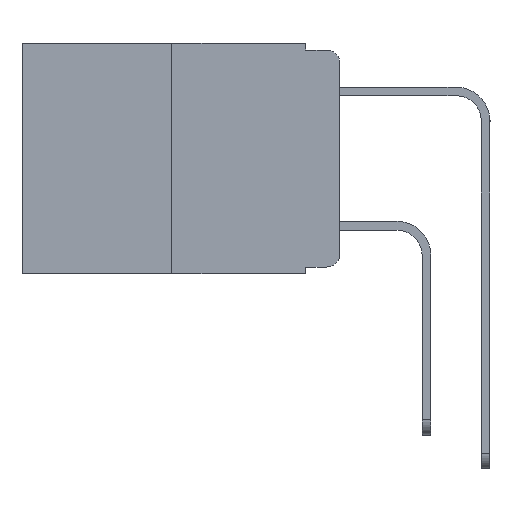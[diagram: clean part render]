
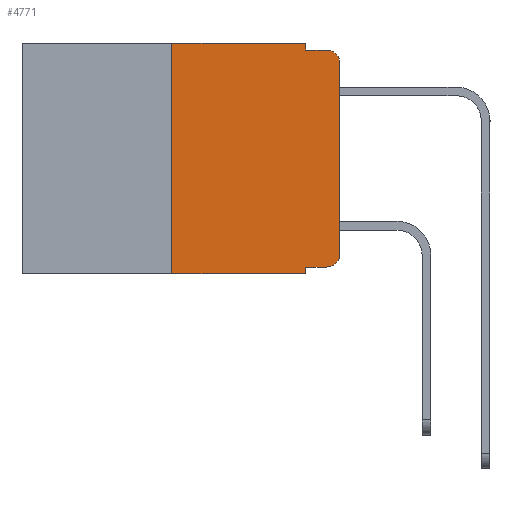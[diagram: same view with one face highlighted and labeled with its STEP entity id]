
A CAD part, left-side view. The second image highlights one B-rep face of the part: STEP entity #4771.
In plain terms, the highlighted planar face has unit normal (-1, 0, 0).
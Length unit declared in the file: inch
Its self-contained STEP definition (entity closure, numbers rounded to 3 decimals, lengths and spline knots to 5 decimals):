
#76 = CARTESIAN_POINT ( 'NONE',  ( 0., 0.473, -0.343 ) ) ;
#360 = VERTEX_POINT ( 'NONE', #22311 ) ;
#963 = VERTEX_POINT ( 'NONE', #10376 ) ;
#1065 = LINE ( 'NONE', #20651, #9861 ) ;
#1160 = DIRECTION ( 'NONE',  ( 0., 0., -1. ) ) ;
#1707 = DIRECTION ( 'NONE',  ( 0., 0., 1. ) ) ;
#1787 = ORIENTED_EDGE ( 'NONE', *, *, #9536, .T. ) ;
#1815 = AXIS2_PLACEMENT_3D ( 'NONE', #21714, #11625, #1160 ) ;
#1966 = CARTESIAN_POINT ( 'NONE',  ( 0., 0.051, -0.333 ) ) ;
#2616 = CARTESIAN_POINT ( 'NONE',  ( 0., 0.02, -0.313 ) ) ;
#2917 = LINE ( 'NONE', #76, #11075 ) ;
#3633 = CARTESIAN_POINT ( 'NONE',  ( 0., 0.051, -0.343 ) ) ;
#3907 = ORIENTED_EDGE ( 'NONE', *, *, #21164, .F. ) ;
#4162 = VERTEX_POINT ( 'NONE', #11497 ) ;
#4263 = VECTOR ( 'NONE', #15003, 39.37008 ) ;
#4376 = DIRECTION ( 'NONE',  ( 0., 0., -1. ) ) ;
#4771 = ADVANCED_FACE ( 'NONE', ( #7834 ), #8651, .F. ) ;
#4985 = ORIENTED_EDGE ( 'NONE', *, *, #8451, .T. ) ;
#5076 = DIRECTION ( 'NONE',  ( 0., -1., 0. ) ) ;
#5082 = EDGE_CURVE ( 'NONE', #963, #19427, #2917, .T. ) ;
#5394 = VECTOR ( 'NONE', #16503, 39.37008 ) ;
#5771 = ORIENTED_EDGE ( 'NONE', *, *, #17593, .F. ) ;
#7051 = AXIS2_PLACEMENT_3D ( 'NONE', #9556, #7081, #12277 ) ;
#7081 = DIRECTION ( 'NONE',  ( 1., 0., 0. ) ) ;
#7834 = FACE_OUTER_BOUND ( 'NONE', #17323, .T. ) ;
#8345 = DIRECTION ( 'NONE',  ( 0., 0., -1. ) ) ;
#8451 = EDGE_CURVE ( 'NONE', #11211, #14397, #16015, .T. ) ;
#8623 = CARTESIAN_POINT ( 'NONE',  ( 0., 0., -0.03 ) ) ;
#8651 = PLANE ( 'NONE',  #7051 ) ;
#8987 = ORIENTED_EDGE ( 'NONE', *, *, #20692, .F. ) ;
#9296 = ORIENTED_EDGE ( 'NONE', *, *, #20279, .F. ) ;
#9536 = EDGE_CURVE ( 'NONE', #360, #19027, #14230, .T. ) ;
#9556 = CARTESIAN_POINT ( 'NONE',  ( 0., 0.473, 0. ) ) ;
#9861 = VECTOR ( 'NONE', #22258, 39.37008 ) ;
#10049 = VECTOR ( 'NONE', #15647, 39.37008 ) ;
#10376 = CARTESIAN_POINT ( 'NONE',  ( 0., 0.25, -0.343 ) ) ;
#10424 = LINE ( 'NONE', #12122, #19985 ) ;
#10540 = LINE ( 'NONE', #13305, #4263 ) ;
#10588 = LINE ( 'NONE', #22256, #10049 ) ;
#10656 = DIRECTION ( 'NONE',  ( 0., -1., 0. ) ) ;
#11075 = VECTOR ( 'NONE', #10656, 39.37008 ) ;
#11211 = VERTEX_POINT ( 'NONE', #8623 ) ;
#11252 = CARTESIAN_POINT ( 'NONE',  ( 0., 0., -0.313 ) ) ;
#11497 = CARTESIAN_POINT ( 'NONE',  ( 0., 0.051, -0.01 ) ) ;
#11625 = DIRECTION ( 'NONE',  ( -1., 0., 0. ) ) ;
#11812 = CARTESIAN_POINT ( 'NONE',  ( 0., 0.051, 0. ) ) ;
#11914 = EDGE_CURVE ( 'NONE', #19027, #11211, #1065, .T. ) ;
#12122 = CARTESIAN_POINT ( 'NONE',  ( 0., 0.25, 0. ) ) ;
#12277 = DIRECTION ( 'NONE',  ( 0., 0., -1. ) ) ;
#12385 = CARTESIAN_POINT ( 'NONE',  ( 0., 0.051, 0. ) ) ;
#12521 = LINE ( 'NONE', #11812, #15441 ) ;
#12955 = CARTESIAN_POINT ( 'NONE',  ( 0., 0.02, -0.01 ) ) ;
#12986 = EDGE_CURVE ( 'NONE', #14159, #19427, #12521, .T. ) ;
#13305 = CARTESIAN_POINT ( 'NONE',  ( 0., 0.051, 0. ) ) ;
#13616 = AXIS2_PLACEMENT_3D ( 'NONE', #2616, #14708, #4376 ) ;
#14044 = VECTOR ( 'NONE', #5076, 39.37008 ) ;
#14114 = EDGE_CURVE ( 'NONE', #14159, #360, #10588, .T. ) ;
#14159 = VERTEX_POINT ( 'NONE', #1966 ) ;
#14230 = CIRCLE ( 'NONE', #13616, 0.02 ) ;
#14397 = VERTEX_POINT ( 'NONE', #12955 ) ;
#14551 = LINE ( 'NONE', #18238, #5394 ) ;
#14708 = DIRECTION ( 'NONE',  ( -1., 0., 0. ) ) ;
#15003 = DIRECTION ( 'NONE',  ( 0., 0., -1. ) ) ;
#15019 = ORIENTED_EDGE ( 'NONE', *, *, #12986, .F. ) ;
#15441 = VECTOR ( 'NONE', #8345, 39.37008 ) ;
#15647 = DIRECTION ( 'NONE',  ( 0., -1., 0. ) ) ;
#15650 = LINE ( 'NONE', #20462, #14044 ) ;
#16015 = CIRCLE ( 'NONE', #1815, 0.02 ) ;
#16503 = DIRECTION ( 'NONE',  ( 0., -1., 0. ) ) ;
#16780 = ORIENTED_EDGE ( 'NONE', *, *, #11914, .T. ) ;
#17060 = VERTEX_POINT ( 'NONE', #12385 ) ;
#17323 = EDGE_LOOP ( 'NONE', ( #16780, #4985, #9296, #3907, #8987, #5771, #17392, #15019, #17517, #1787 ) ) ;
#17392 = ORIENTED_EDGE ( 'NONE', *, *, #5082, .T. ) ;
#17517 = ORIENTED_EDGE ( 'NONE', *, *, #14114, .T. ) ;
#17593 = EDGE_CURVE ( 'NONE', #963, #21235, #10424, .T. ) ;
#18238 = CARTESIAN_POINT ( 'NONE',  ( 0., 0.473, 0. ) ) ;
#18696 = CARTESIAN_POINT ( 'NONE',  ( 0., 0.25, 0. ) ) ;
#19027 = VERTEX_POINT ( 'NONE', #11252 ) ;
#19427 = VERTEX_POINT ( 'NONE', #3633 ) ;
#19985 = VECTOR ( 'NONE', #1707, 39.37008 ) ;
#20279 = EDGE_CURVE ( 'NONE', #4162, #14397, #15650, .T. ) ;
#20462 = CARTESIAN_POINT ( 'NONE',  ( 0., 0.051, -0.01 ) ) ;
#20651 = CARTESIAN_POINT ( 'NONE',  ( 0., 0., 0. ) ) ;
#20692 = EDGE_CURVE ( 'NONE', #21235, #17060, #14551, .T. ) ;
#21164 = EDGE_CURVE ( 'NONE', #17060, #4162, #10540, .T. ) ;
#21235 = VERTEX_POINT ( 'NONE', #18696 ) ;
#21714 = CARTESIAN_POINT ( 'NONE',  ( 0., 0.02, -0.03 ) ) ;
#22256 = CARTESIAN_POINT ( 'NONE',  ( 0., 0.051, -0.333 ) ) ;
#22258 = DIRECTION ( 'NONE',  ( 0., 0., 1. ) ) ;
#22311 = CARTESIAN_POINT ( 'NONE',  ( 0., 0.02, -0.333 ) ) ;
